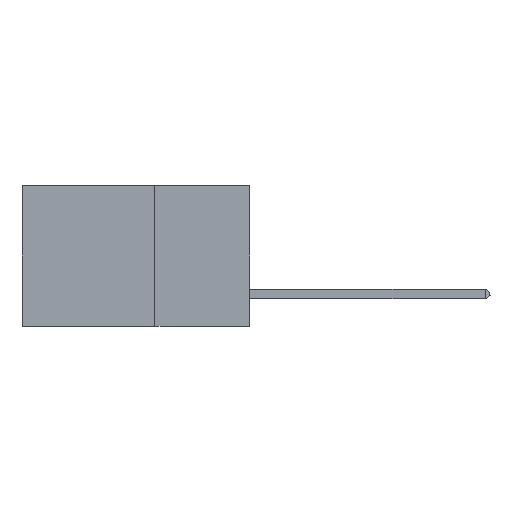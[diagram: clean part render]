
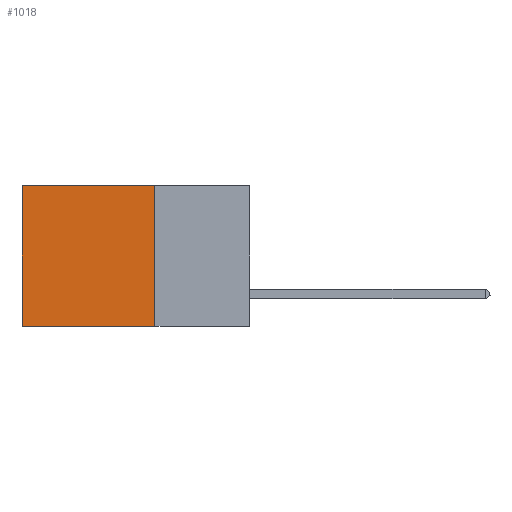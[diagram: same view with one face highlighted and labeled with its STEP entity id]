
A CAD part, left-side view. The second image highlights one B-rep face of the part: STEP entity #1018.
In plain terms, the highlighted planar face has unit normal (-1, 0, 0).
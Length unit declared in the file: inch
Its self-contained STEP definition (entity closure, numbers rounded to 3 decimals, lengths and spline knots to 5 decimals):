
#592 = CARTESIAN_POINT ( 'NONE',  ( 0.2875, 0.25, 0. ) ) ;
#1018 = ADVANCED_FACE ( 'NONE', ( #1532 ), #7316, .F. ) ;
#1427 = DIRECTION ( 'NONE',  ( 1., 0., 0. ) ) ;
#1532 = FACE_OUTER_BOUND ( 'NONE', #19231, .T. ) ;
#2648 = CARTESIAN_POINT ( 'NONE',  ( 0.2875, 0.25, -0.37 ) ) ;
#3280 = CARTESIAN_POINT ( 'NONE',  ( 0.2875, 0.25, -0.37 ) ) ;
#3597 = VERTEX_POINT ( 'NONE', #27765 ) ;
#4091 = EDGE_CURVE ( 'NONE', #16808, #7243, #13098, .T. ) ;
#4959 = DIRECTION ( 'NONE',  ( 0., 0., -1. ) ) ;
#6257 = VECTOR ( 'NONE', #14095, 39.37008 ) ;
#7001 = LINE ( 'NONE', #592, #9354 ) ;
#7117 = DIRECTION ( 'NONE',  ( 0., 1., 0. ) ) ;
#7243 = VERTEX_POINT ( 'NONE', #2648 ) ;
#7316 = PLANE ( 'NONE',  #16945 ) ;
#7471 = EDGE_CURVE ( 'NONE', #3597, #27235, #14103, .T. ) ;
#8743 = VECTOR ( 'NONE', #4959, 39.37008 ) ;
#9354 = VECTOR ( 'NONE', #7117, 39.37008 ) ;
#9739 = CARTESIAN_POINT ( 'NONE',  ( 0.2875, 0.25, 0. ) ) ;
#10019 = CARTESIAN_POINT ( 'NONE',  ( 0.2875, 0.25, 0. ) ) ;
#10899 = ORIENTED_EDGE ( 'NONE', *, *, #4091, .F. ) ;
#11529 = CARTESIAN_POINT ( 'NONE',  ( 0.2875, 0.25, 0. ) ) ;
#11661 = ORIENTED_EDGE ( 'NONE', *, *, #7471, .T. ) ;
#13098 = LINE ( 'NONE', #11529, #23561 ) ;
#13467 = DIRECTION ( 'NONE',  ( 0., 0., -1. ) ) ;
#14095 = DIRECTION ( 'NONE',  ( 0., 1., 0. ) ) ;
#14103 = LINE ( 'NONE', #17385, #8743 ) ;
#16808 = VERTEX_POINT ( 'NONE', #9739 ) ;
#16945 = AXIS2_PLACEMENT_3D ( 'NONE', #10019, #1427, #24854 ) ;
#17043 = EDGE_CURVE ( 'NONE', #7243, #27235, #23076, .T. ) ;
#17385 = CARTESIAN_POINT ( 'NONE',  ( 0.2875, 0.6, 0. ) ) ;
#18027 = ORIENTED_EDGE ( 'NONE', *, *, #22202, .T. ) ;
#19231 = EDGE_LOOP ( 'NONE', ( #11661, #21526, #10899, #18027 ) ) ;
#21526 = ORIENTED_EDGE ( 'NONE', *, *, #17043, .F. ) ;
#22202 = EDGE_CURVE ( 'NONE', #16808, #3597, #7001, .T. ) ;
#22661 = CARTESIAN_POINT ( 'NONE',  ( 0.2875, 0.6, -0.37 ) ) ;
#23076 = LINE ( 'NONE', #3280, #6257 ) ;
#23561 = VECTOR ( 'NONE', #13467, 39.37008 ) ;
#24854 = DIRECTION ( 'NONE',  ( 0., 0., -1. ) ) ;
#27235 = VERTEX_POINT ( 'NONE', #22661 ) ;
#27765 = CARTESIAN_POINT ( 'NONE',  ( 0.2875, 0.6, 0. ) ) ;
